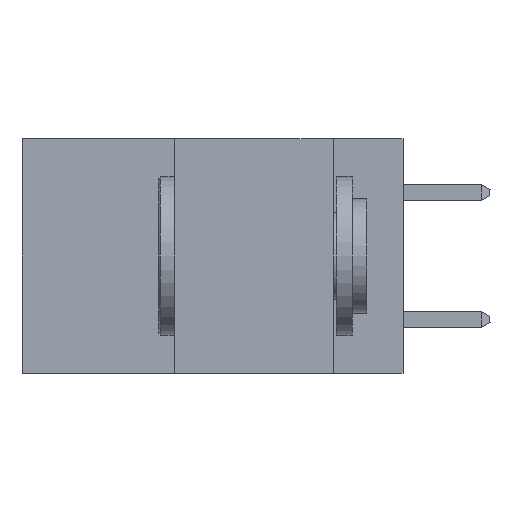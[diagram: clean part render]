
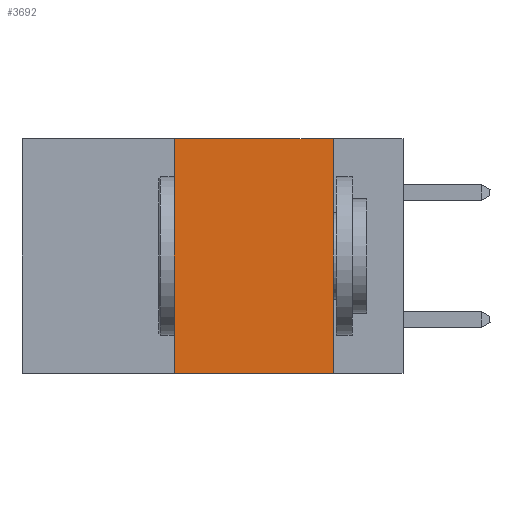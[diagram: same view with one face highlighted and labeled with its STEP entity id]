
A CAD part, left-side view. The second image highlights one B-rep face of the part: STEP entity #3692.
In plain terms, the highlighted planar face has unit normal (-1, 0, 0).
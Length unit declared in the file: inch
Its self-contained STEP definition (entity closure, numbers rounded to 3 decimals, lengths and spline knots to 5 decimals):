
#732 = VERTEX_POINT ( 'NONE', #2631 ) ;
#901 = VERTEX_POINT ( 'NONE', #13221 ) ;
#1567 = CARTESIAN_POINT ( 'NONE',  ( 0., 0.11, 0. ) ) ;
#1929 = CARTESIAN_POINT ( 'NONE',  ( 0., 0.36, 0. ) ) ;
#2631 = CARTESIAN_POINT ( 'NONE',  ( 0., 0.36, -0.37 ) ) ;
#3046 = EDGE_LOOP ( 'NONE', ( #24078, #12855, #12546, #12025 ) ) ;
#3143 = DIRECTION ( 'NONE',  ( 0., -1., 0. ) ) ;
#3564 = EDGE_CURVE ( 'NONE', #732, #13827, #8053, .T. ) ;
#3692 = ADVANCED_FACE ( 'NONE', ( #17187 ), #25321, .F. ) ;
#4040 = EDGE_CURVE ( 'NONE', #732, #24893, #13900, .T. ) ;
#5983 = DIRECTION ( 'NONE',  ( 0., -1., 0. ) ) ;
#7378 = VECTOR ( 'NONE', #5983, 39.37008 ) ;
#8053 = LINE ( 'NONE', #12228, #7378 ) ;
#9332 = CARTESIAN_POINT ( 'NONE',  ( 0., 0.6, 0. ) ) ;
#12025 = ORIENTED_EDGE ( 'NONE', *, *, #3564, .T. ) ;
#12228 = CARTESIAN_POINT ( 'NONE',  ( 0., 0.6, -0.37 ) ) ;
#12524 = DIRECTION ( 'NONE',  ( 0., 0., -1. ) ) ;
#12546 = ORIENTED_EDGE ( 'NONE', *, *, #4040, .F. ) ;
#12855 = ORIENTED_EDGE ( 'NONE', *, *, #14691, .F. ) ;
#13221 = CARTESIAN_POINT ( 'NONE',  ( 0., 0.11, 0. ) ) ;
#13827 = VERTEX_POINT ( 'NONE', #16998 ) ;
#13900 = LINE ( 'NONE', #15842, #20151 ) ;
#14691 = EDGE_CURVE ( 'NONE', #24893, #901, #18486, .T. ) ;
#14850 = EDGE_CURVE ( 'NONE', #901, #13827, #17119, .T. ) ;
#15842 = CARTESIAN_POINT ( 'NONE',  ( 0., 0.36, 0. ) ) ;
#16998 = CARTESIAN_POINT ( 'NONE',  ( 0., 0.11, -0.37 ) ) ;
#17119 = LINE ( 'NONE', #1567, #20425 ) ;
#17187 = FACE_OUTER_BOUND ( 'NONE', #3046, .T. ) ;
#18486 = LINE ( 'NONE', #9332, #25057 ) ;
#18952 = DIRECTION ( 'NONE',  ( 1., 0., 0. ) ) ;
#20151 = VECTOR ( 'NONE', #23930, 39.37008 ) ;
#20425 = VECTOR ( 'NONE', #22534, 39.37008 ) ;
#20883 = AXIS2_PLACEMENT_3D ( 'NONE', #25043, #18952, #12524 ) ;
#22534 = DIRECTION ( 'NONE',  ( 0., 0., -1. ) ) ;
#23930 = DIRECTION ( 'NONE',  ( 0., 0., 1. ) ) ;
#24078 = ORIENTED_EDGE ( 'NONE', *, *, #14850, .F. ) ;
#24893 = VERTEX_POINT ( 'NONE', #1929 ) ;
#25043 = CARTESIAN_POINT ( 'NONE',  ( 0., 0.6, 0. ) ) ;
#25057 = VECTOR ( 'NONE', #3143, 39.37008 ) ;
#25321 = PLANE ( 'NONE',  #20883 ) ;
